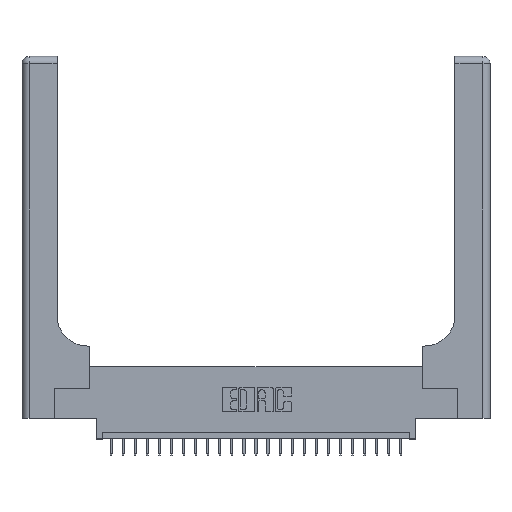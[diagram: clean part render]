
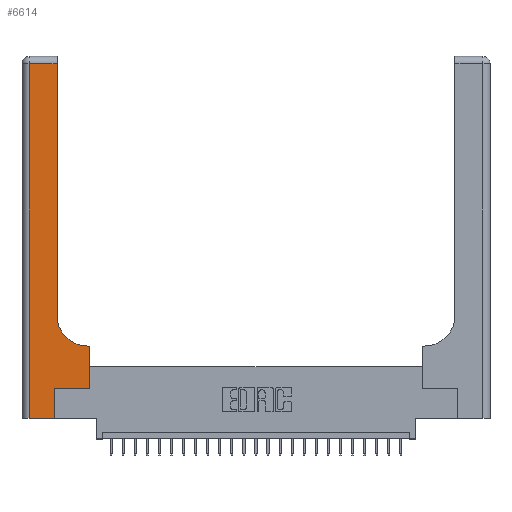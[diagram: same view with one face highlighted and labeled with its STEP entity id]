
A CAD part, top view. The second image highlights one B-rep face of the part: STEP entity #6614.
In plain terms, the highlighted planar face has unit normal (0, 0, 1).
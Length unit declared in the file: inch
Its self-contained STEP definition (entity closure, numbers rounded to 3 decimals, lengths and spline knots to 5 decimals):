
#49 = ORIENTED_EDGE ( 'NONE', *, *, #13261, .T. ) ;
#506 = EDGE_LOOP ( 'NONE', ( #5228, #9923, #15409, #49, #26012, #20073, #12700, #5950, #26478 ) ) ;
#526 = CARTESIAN_POINT ( 'NONE',  ( 0.5415, 0.6, 0.37 ) ) ;
#612 = CARTESIAN_POINT ( 'NONE',  ( 0.06, 0., 0.37 ) ) ;
#1053 = CIRCLE ( 'NONE', #23766, 0.25 ) ;
#1669 = VECTOR ( 'NONE', #20028, 39.37008 ) ;
#1675 = EDGE_CURVE ( 'NONE', #17108, #4613, #15254, .T. ) ;
#2883 = DIRECTION ( 'NONE',  ( 1., 0., 0. ) ) ;
#3057 = VECTOR ( 'NONE', #7095, 39.37008 ) ;
#4613 = VERTEX_POINT ( 'NONE', #526 ) ;
#5064 = DIRECTION ( 'NONE',  ( -1., 0., 0. ) ) ;
#5228 = ORIENTED_EDGE ( 'NONE', *, *, #14565, .T. ) ;
#5564 = CARTESIAN_POINT ( 'NONE',  ( 0.06, 2.94, 0.37 ) ) ;
#5950 = ORIENTED_EDGE ( 'NONE', *, *, #1675, .T. ) ;
#6614 = ADVANCED_FACE ( 'NONE', ( #13957 ), #9933, .F. ) ;
#7095 = DIRECTION ( 'NONE',  ( 0., 1., 0. ) ) ;
#7710 = CARTESIAN_POINT ( 'NONE',  ( 0.269, 0.25, 0.37 ) ) ;
#7937 = VECTOR ( 'NONE', #2883, 39.37008 ) ;
#8613 = CARTESIAN_POINT ( 'NONE',  ( 0.269, 0.25, 0.37 ) ) ;
#8939 = LINE ( 'NONE', #23127, #15244 ) ;
#9813 = VERTEX_POINT ( 'NONE', #23142 ) ;
#9923 = ORIENTED_EDGE ( 'NONE', *, *, #26255, .T. ) ;
#9933 = PLANE ( 'NONE',  #21856 ) ;
#10146 = DIRECTION ( 'NONE',  ( 1., 0., 0. ) ) ;
#10237 = VERTEX_POINT ( 'NONE', #16960 ) ;
#10447 = LINE ( 'NONE', #14866, #23377 ) ;
#10764 = CARTESIAN_POINT ( 'NONE',  ( 0.269, 0., 0.37 ) ) ;
#10834 = LINE ( 'NONE', #17005, #3057 ) ;
#11121 = EDGE_CURVE ( 'NONE', #4613, #10237, #1053, .T. ) ;
#11206 = VERTEX_POINT ( 'NONE', #612 ) ;
#11942 = DIRECTION ( 'NONE',  ( 0., 0., -1. ) ) ;
#11992 = LINE ( 'NONE', #7710, #1669 ) ;
#12196 = CARTESIAN_POINT ( 'NONE',  ( 0.5585, 0.25, 0.37 ) ) ;
#12700 = ORIENTED_EDGE ( 'NONE', *, *, #19557, .T. ) ;
#13261 = EDGE_CURVE ( 'NONE', #11206, #25078, #25151, .T. ) ;
#13423 = VECTOR ( 'NONE', #5064, 39.37008 ) ;
#13957 = FACE_OUTER_BOUND ( 'NONE', #506, .T. ) ;
#14565 = EDGE_CURVE ( 'NONE', #10237, #9813, #10447, .T. ) ;
#14656 = LINE ( 'NONE', #22573, #23660 ) ;
#14866 = CARTESIAN_POINT ( 'NONE',  ( 0.2915, 3., 0.37 ) ) ;
#15244 = VECTOR ( 'NONE', #16840, 39.37008 ) ;
#15254 = LINE ( 'NONE', #23426, #13423 ) ;
#15409 = ORIENTED_EDGE ( 'NONE', *, *, #16040, .T. ) ;
#15675 = LINE ( 'NONE', #19161, #16591 ) ;
#15704 = CARTESIAN_POINT ( 'NONE',  ( 0., 3., 0.37 ) ) ;
#16040 = EDGE_CURVE ( 'NONE', #26511, #11206, #15675, .T. ) ;
#16591 = VECTOR ( 'NONE', #21707, 39.37008 ) ;
#16840 = DIRECTION ( 'NONE',  ( -1., 0., 0. ) ) ;
#16960 = CARTESIAN_POINT ( 'NONE',  ( 0.2915, 0.85, 0.37 ) ) ;
#17005 = CARTESIAN_POINT ( 'NONE',  ( 0.5585, 0.25, 0.37 ) ) ;
#17108 = VERTEX_POINT ( 'NONE', #22831 ) ;
#18407 = EDGE_CURVE ( 'NONE', #18991, #21857, #11992, .T. ) ;
#18608 = DIRECTION ( 'NONE',  ( 0., 1., 0. ) ) ;
#18991 = VERTEX_POINT ( 'NONE', #8613 ) ;
#19161 = CARTESIAN_POINT ( 'NONE',  ( 0.06, 3., 0.37 ) ) ;
#19557 = EDGE_CURVE ( 'NONE', #21857, #17108, #10834, .T. ) ;
#20028 = DIRECTION ( 'NONE',  ( 1., 0., 0. ) ) ;
#20073 = ORIENTED_EDGE ( 'NONE', *, *, #18407, .T. ) ;
#20100 = DIRECTION ( 'NONE',  ( -1., 0., 0. ) ) ;
#20942 = EDGE_CURVE ( 'NONE', #25078, #18991, #14656, .T. ) ;
#21707 = DIRECTION ( 'NONE',  ( 0., -1., 0. ) ) ;
#21856 = AXIS2_PLACEMENT_3D ( 'NONE', #15704, #11942, #20100 ) ;
#21857 = VERTEX_POINT ( 'NONE', #12196 ) ;
#22573 = CARTESIAN_POINT ( 'NONE',  ( 0.269, 0., 0.37 ) ) ;
#22695 = DIRECTION ( 'NONE',  ( 0., 1., 0. ) ) ;
#22831 = CARTESIAN_POINT ( 'NONE',  ( 0.5585, 0.6, 0.37 ) ) ;
#23127 = CARTESIAN_POINT ( 'NONE',  ( 0., 2.94, 0.37 ) ) ;
#23142 = CARTESIAN_POINT ( 'NONE',  ( 0.2915, 2.94, 0.37 ) ) ;
#23377 = VECTOR ( 'NONE', #18608, 39.37008 ) ;
#23426 = CARTESIAN_POINT ( 'NONE',  ( 0.2915, 0.6, 0.37 ) ) ;
#23660 = VECTOR ( 'NONE', #22695, 39.37008 ) ;
#23766 = AXIS2_PLACEMENT_3D ( 'NONE', #26236, #24217, #10146 ) ;
#24217 = DIRECTION ( 'NONE',  ( 0., 0., -1. ) ) ;
#25078 = VERTEX_POINT ( 'NONE', #10764 ) ;
#25151 = LINE ( 'NONE', #25272, #7937 ) ;
#25272 = CARTESIAN_POINT ( 'NONE',  ( 0., 0., 0.37 ) ) ;
#26012 = ORIENTED_EDGE ( 'NONE', *, *, #20942, .T. ) ;
#26236 = CARTESIAN_POINT ( 'NONE',  ( 0.5415, 0.85, 0.37 ) ) ;
#26255 = EDGE_CURVE ( 'NONE', #9813, #26511, #8939, .T. ) ;
#26478 = ORIENTED_EDGE ( 'NONE', *, *, #11121, .T. ) ;
#26511 = VERTEX_POINT ( 'NONE', #5564 ) ;
